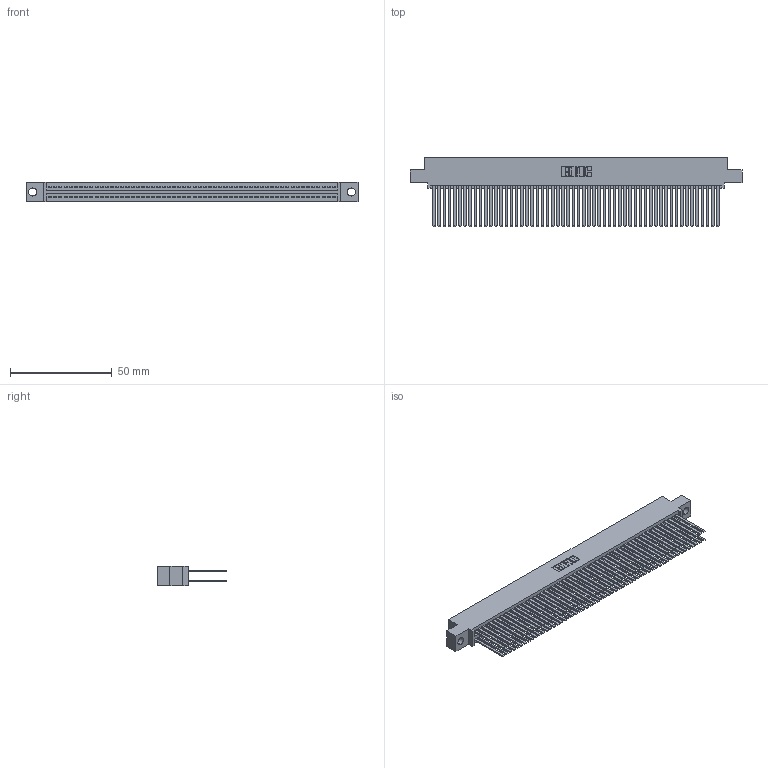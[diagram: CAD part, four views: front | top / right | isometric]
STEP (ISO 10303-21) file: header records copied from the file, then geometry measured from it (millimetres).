
FILE_DESCRIPTION (( 'STEP AP203' ), '1' );
FILE_NAME ('345-112-544-504.STEP', '2021-05-25T14:35:05', ( '' ), ( '' ), 'SwSTEP 2.0', 'SolidWorks 2020', '' );
FILE_SCHEMA (( 'CONFIG_CONTROL_DESIGN' ));
Length unit declared in the file: inch
Products named in the file (3): 345-292-001_345-293-144; 345 Part_0.110 Offset - 0.156 Dia-TI; 345-112-544-504
Assembly tree (113 placements, depth 2):
  345-112-544-504
    345 Part_0.110 Offset - 0.156 Dia-TI
    345-292-001_345-293-144  x112
Bounding box: 163.45 x 33.96 x 9.4 mm (x, y, z)
Volume: 17398.3 mm3; surface area: 30534.8 mm2
Topology: 113 solids, 113 shells, 5072 faces, 15061 edges, 9890 vertices
Faces by surface type: plane 3346, cylinder 1726
Entity records: 42421 total; most frequent: CARTESIAN_POINT 7102, ORIENTED_EDGE 7034, DIRECTION 6241, EDGE_CURVE 3517, VECTOR 3165, LINE 3165, VERTEX_POINT 2342, AXIS2_PLACEMENT_3D 1538
